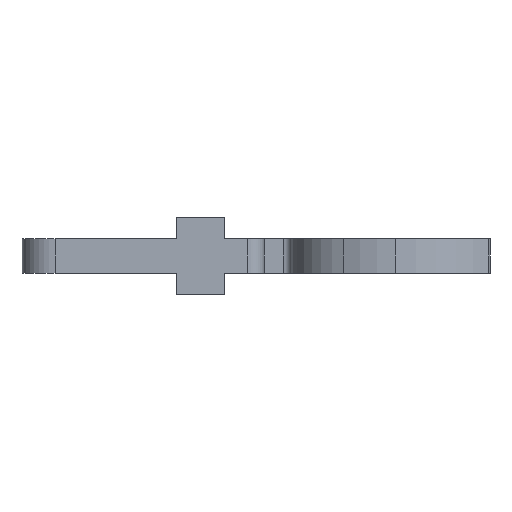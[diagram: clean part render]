
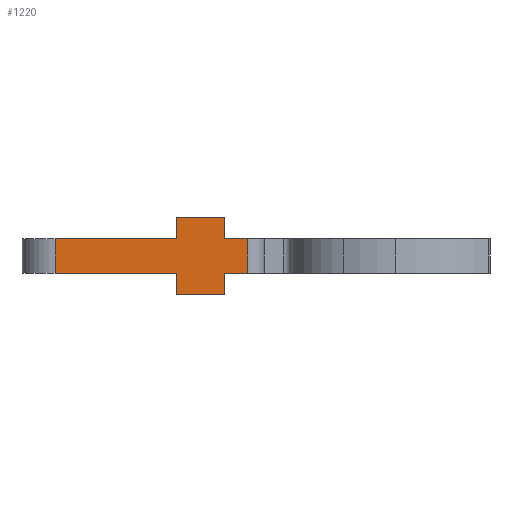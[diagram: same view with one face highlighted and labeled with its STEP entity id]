
A CAD part, left-side view. The second image highlights one B-rep face of the part: STEP entity #1220.
In plain terms, the highlighted planar face has unit normal (-1, 0, 0).
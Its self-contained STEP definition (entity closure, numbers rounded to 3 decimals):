
#2 = ORIENTED_EDGE ( 'NONE', *, *, #1111, .F. ) ;
#9 = LINE ( 'NONE', #496, #652 ) ;
#10 = CARTESIAN_POINT ( 'NONE',  ( 0., 8.382, 0. ) ) ;
#20 = PLANE ( 'NONE',  #747 ) ;
#28 = DIRECTION ( 'NONE',  ( 0., 1., 0. ) ) ;
#42 = CARTESIAN_POINT ( 'NONE',  ( 0., 8.382, 3.302 ) ) ;
#45 = LINE ( 'NONE', #1270, #1358 ) ;
#47 = LINE ( 'NONE', #521, #210 ) ;
#62 = LINE ( 'NONE', #1538, #107 ) ;
#97 = CARTESIAN_POINT ( 'NONE',  ( 0., 1.587, 3.302 ) ) ;
#107 = VECTOR ( 'NONE', #941, 1000. ) ;
#110 = VECTOR ( 'NONE', #1435, 1000. ) ;
#161 = CARTESIAN_POINT ( 'NONE',  ( 0., 20.066, 3.302 ) ) ;
#168 = LINE ( 'NONE', #356, #811 ) ;
#210 = VECTOR ( 'NONE', #479, 1000. ) ;
#223 = ORIENTED_EDGE ( 'NONE', *, *, #525, .F. ) ;
#233 = VECTOR ( 'NONE', #886, 1000. ) ;
#235 = CARTESIAN_POINT ( 'NONE',  ( 0., 23.241, 3.302 ) ) ;
#239 = CARTESIAN_POINT ( 'NONE',  ( 0., 3.81, 5.334 ) ) ;
#248 = VECTOR ( 'NONE', #1262, 1000. ) ;
#252 = VERTEX_POINT ( 'NONE', #1365 ) ;
#264 = ORIENTED_EDGE ( 'NONE', *, *, #817, .T. ) ;
#289 = DIRECTION ( 'NONE',  ( 0., 0., 1. ) ) ;
#308 = CARTESIAN_POINT ( 'NONE',  ( 0., 3.81, 3.302 ) ) ;
#327 = CARTESIAN_POINT ( 'NONE',  ( 0., 3.81, -2.032 ) ) ;
#333 = CARTESIAN_POINT ( 'NONE',  ( 0., 20.066, 3.302 ) ) ;
#354 = VERTEX_POINT ( 'NONE', #1164 ) ;
#356 = CARTESIAN_POINT ( 'NONE',  ( 0., 23.241, 3.302 ) ) ;
#372 = DIRECTION ( 'NONE',  ( 0., 0., 1. ) ) ;
#381 = EDGE_CURVE ( 'NONE', #252, #1296, #47, .T. ) ;
#394 = ORIENTED_EDGE ( 'NONE', *, *, #381, .T. ) ;
#405 = EDGE_CURVE ( 'NONE', #812, #773, #168, .T. ) ;
#413 = CARTESIAN_POINT ( 'NONE',  ( 0., 23.241, 3.302 ) ) ;
#434 = DIRECTION ( 'NONE',  ( 0., 0., -1. ) ) ;
#457 = DIRECTION ( 'NONE',  ( 0., -1., 0. ) ) ;
#467 = LINE ( 'NONE', #235, #248 ) ;
#479 = DIRECTION ( 'NONE',  ( 0., 0., -1. ) ) ;
#491 = EDGE_CURVE ( 'NONE', #1096, #898, #9, .T. ) ;
#496 = CARTESIAN_POINT ( 'NONE',  ( 0., 23.241, 0. ) ) ;
#499 = EDGE_CURVE ( 'NONE', #354, #940, #692, .T. ) ;
#521 = CARTESIAN_POINT ( 'NONE',  ( 0., 8.382, 5.334 ) ) ;
#525 = EDGE_CURVE ( 'NONE', #717, #712, #1257, .T. ) ;
#553 = EDGE_CURVE ( 'NONE', #879, #1096, #574, .T. ) ;
#574 = LINE ( 'NONE', #333, #1176 ) ;
#584 = CARTESIAN_POINT ( 'NONE',  ( 0., 1.587, 3.302 ) ) ;
#590 = LINE ( 'NONE', #97, #971 ) ;
#606 = EDGE_CURVE ( 'NONE', #252, #1080, #754, .T. ) ;
#652 = VECTOR ( 'NONE', #1475, 1000. ) ;
#692 = LINE ( 'NONE', #1581, #954 ) ;
#712 = VERTEX_POINT ( 'NONE', #979 ) ;
#717 = VERTEX_POINT ( 'NONE', #964 ) ;
#747 = AXIS2_PLACEMENT_3D ( 'NONE', #413, #797, #28 ) ;
#754 = LINE ( 'NONE', #1457, #110 ) ;
#773 = VERTEX_POINT ( 'NONE', #584 ) ;
#797 = DIRECTION ( 'NONE',  ( 1., 0., 0. ) ) ;
#811 = VECTOR ( 'NONE', #457, 1000. ) ;
#812 = VERTEX_POINT ( 'NONE', #308 ) ;
#817 = EDGE_CURVE ( 'NONE', #717, #354, #1287, .T. ) ;
#879 = VERTEX_POINT ( 'NONE', #161 ) ;
#886 = DIRECTION ( 'NONE',  ( 0., 1., 0. ) ) ;
#898 = VERTEX_POINT ( 'NONE', #10 ) ;
#940 = VERTEX_POINT ( 'NONE', #1228 ) ;
#941 = DIRECTION ( 'NONE',  ( 0., 0., -1. ) ) ;
#954 = VECTOR ( 'NONE', #1361, 1000. ) ;
#964 = CARTESIAN_POINT ( 'NONE',  ( 0., 3.81, -2.032 ) ) ;
#971 = VECTOR ( 'NONE', #987, 1000. ) ;
#979 = CARTESIAN_POINT ( 'NONE',  ( 0., 8.382, -2.032 ) ) ;
#987 = DIRECTION ( 'NONE',  ( 0., 0., 1. ) ) ;
#991 = CARTESIAN_POINT ( 'NONE',  ( 0., 8.382, -2.032 ) ) ;
#1005 = EDGE_CURVE ( 'NONE', #940, #773, #590, .T. ) ;
#1010 = ORIENTED_EDGE ( 'NONE', *, *, #1065, .F. ) ;
#1012 = CARTESIAN_POINT ( 'NONE',  ( 0., 20.066, 0. ) ) ;
#1065 = EDGE_CURVE ( 'NONE', #879, #1296, #467, .T. ) ;
#1080 = VERTEX_POINT ( 'NONE', #239 ) ;
#1096 = VERTEX_POINT ( 'NONE', #1012 ) ;
#1111 = EDGE_CURVE ( 'NONE', #712, #898, #45, .T. ) ;
#1117 = EDGE_LOOP ( 'NONE', ( #1595, #1550, #1555, #1144, #1554, #394, #1010, #1572, #1613, #2, #223, #264 ) ) ;
#1144 = ORIENTED_EDGE ( 'NONE', *, *, #1263, .F. ) ;
#1164 = CARTESIAN_POINT ( 'NONE',  ( 0., 3.81, 0. ) ) ;
#1171 = FACE_OUTER_BOUND ( 'NONE', #1117, .T. ) ;
#1176 = VECTOR ( 'NONE', #434, 1000. ) ;
#1220 = ADVANCED_FACE ( 'NONE', ( #1171 ), #20, .F. ) ;
#1228 = CARTESIAN_POINT ( 'NONE',  ( 0., 1.587, 0. ) ) ;
#1257 = LINE ( 'NONE', #991, #233 ) ;
#1262 = DIRECTION ( 'NONE',  ( 0., -1., 0. ) ) ;
#1263 = EDGE_CURVE ( 'NONE', #1080, #812, #62, .T. ) ;
#1270 = CARTESIAN_POINT ( 'NONE',  ( 0., 8.382, -2.032 ) ) ;
#1287 = LINE ( 'NONE', #327, #1548 ) ;
#1296 = VERTEX_POINT ( 'NONE', #42 ) ;
#1358 = VECTOR ( 'NONE', #372, 1000. ) ;
#1361 = DIRECTION ( 'NONE',  ( 0., -1., 0. ) ) ;
#1365 = CARTESIAN_POINT ( 'NONE',  ( 0., 8.382, 5.334 ) ) ;
#1435 = DIRECTION ( 'NONE',  ( 0., -1., 0. ) ) ;
#1457 = CARTESIAN_POINT ( 'NONE',  ( 0., 3.81, 5.334 ) ) ;
#1475 = DIRECTION ( 'NONE',  ( 0., -1., 0. ) ) ;
#1538 = CARTESIAN_POINT ( 'NONE',  ( 0., 3.81, 5.334 ) ) ;
#1548 = VECTOR ( 'NONE', #289, 1000. ) ;
#1550 = ORIENTED_EDGE ( 'NONE', *, *, #1005, .T. ) ;
#1554 = ORIENTED_EDGE ( 'NONE', *, *, #606, .F. ) ;
#1555 = ORIENTED_EDGE ( 'NONE', *, *, #405, .F. ) ;
#1572 = ORIENTED_EDGE ( 'NONE', *, *, #553, .T. ) ;
#1581 = CARTESIAN_POINT ( 'NONE',  ( 0., 23.241, 0. ) ) ;
#1595 = ORIENTED_EDGE ( 'NONE', *, *, #499, .T. ) ;
#1613 = ORIENTED_EDGE ( 'NONE', *, *, #491, .T. ) ;
